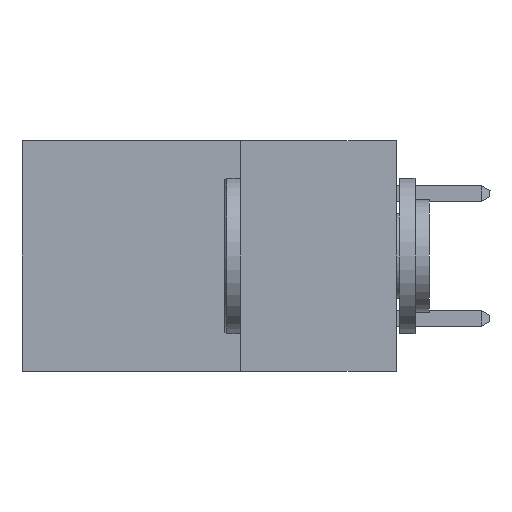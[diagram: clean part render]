
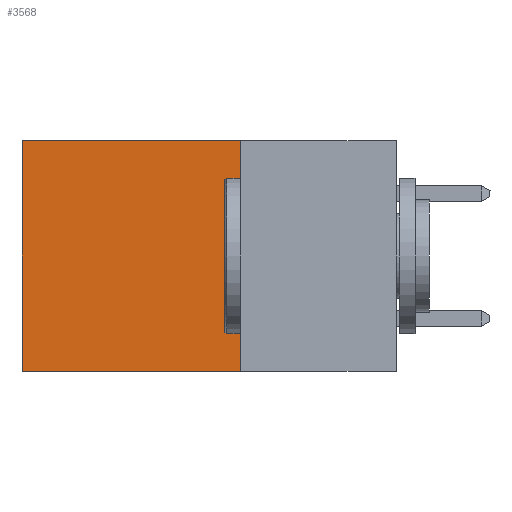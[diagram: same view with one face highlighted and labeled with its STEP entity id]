
A CAD part, left-side view. The second image highlights one B-rep face of the part: STEP entity #3568.
In plain terms, the highlighted planar face has unit normal (-1, 0, 0).
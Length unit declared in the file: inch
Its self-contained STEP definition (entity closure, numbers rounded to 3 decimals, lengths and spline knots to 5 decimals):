
#724 = VERTEX_POINT ( 'NONE', #9673 ) ;
#824 = LINE ( 'NONE', #9982, #15970 ) ;
#1453 = LINE ( 'NONE', #15244, #12769 ) ;
#1887 = EDGE_CURVE ( 'NONE', #4226, #15812, #9149, .T. ) ;
#2807 = VECTOR ( 'NONE', #5515, 39.37008 ) ;
#2882 = PLANE ( 'NONE',  #16731 ) ;
#3568 = ADVANCED_FACE ( 'NONE', ( #10915 ), #2882, .F. ) ;
#4226 = VERTEX_POINT ( 'NONE', #16965 ) ;
#4707 = DIRECTION ( 'NONE',  ( 0., 0., -1. ) ) ;
#5055 = DIRECTION ( 'NONE',  ( 0., 0., -1. ) ) ;
#5515 = DIRECTION ( 'NONE',  ( 0., 1., 0. ) ) ;
#5548 = CARTESIAN_POINT ( 'NONE',  ( 0.298, 0.25, 0. ) ) ;
#5737 = ORIENTED_EDGE ( 'NONE', *, *, #14938, .T. ) ;
#5936 = DIRECTION ( 'NONE',  ( 1., 0., 0. ) ) ;
#6209 = ORIENTED_EDGE ( 'NONE', *, *, #7208, .F. ) ;
#6779 = LINE ( 'NONE', #15608, #2807 ) ;
#7208 = EDGE_CURVE ( 'NONE', #9818, #4226, #824, .T. ) ;
#7973 = ORIENTED_EDGE ( 'NONE', *, *, #13754, .T. ) ;
#8722 = VECTOR ( 'NONE', #17317, 39.37008 ) ;
#9149 = LINE ( 'NONE', #13560, #8722 ) ;
#9673 = CARTESIAN_POINT ( 'NONE',  ( 0.298, 0.6, 0. ) ) ;
#9818 = VERTEX_POINT ( 'NONE', #10135 ) ;
#9982 = CARTESIAN_POINT ( 'NONE',  ( 0.298, 0.25, 0. ) ) ;
#10135 = CARTESIAN_POINT ( 'NONE',  ( 0.298, 0.25, 0. ) ) ;
#10677 = CARTESIAN_POINT ( 'NONE',  ( 0.298, 0.6, -0.37 ) ) ;
#10915 = FACE_OUTER_BOUND ( 'NONE', #18485, .T. ) ;
#12769 = VECTOR ( 'NONE', #5055, 39.37008 ) ;
#13560 = CARTESIAN_POINT ( 'NONE',  ( 0.298, 0.25, -0.37 ) ) ;
#13754 = EDGE_CURVE ( 'NONE', #724, #15812, #1453, .T. ) ;
#14938 = EDGE_CURVE ( 'NONE', #9818, #724, #6779, .T. ) ;
#15244 = CARTESIAN_POINT ( 'NONE',  ( 0.298, 0.6, 0. ) ) ;
#15608 = CARTESIAN_POINT ( 'NONE',  ( 0.298, 0.25, 0. ) ) ;
#15812 = VERTEX_POINT ( 'NONE', #10677 ) ;
#15906 = DIRECTION ( 'NONE',  ( 0., 0., -1. ) ) ;
#15970 = VECTOR ( 'NONE', #4707, 39.37008 ) ;
#16731 = AXIS2_PLACEMENT_3D ( 'NONE', #5548, #5936, #15906 ) ;
#16965 = CARTESIAN_POINT ( 'NONE',  ( 0.298, 0.25, -0.37 ) ) ;
#17302 = ORIENTED_EDGE ( 'NONE', *, *, #1887, .F. ) ;
#17317 = DIRECTION ( 'NONE',  ( 0., 1., 0. ) ) ;
#18485 = EDGE_LOOP ( 'NONE', ( #7973, #17302, #6209, #5737 ) ) ;
